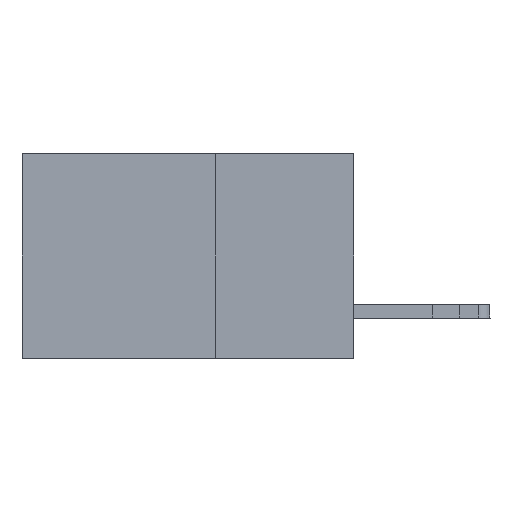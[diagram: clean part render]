
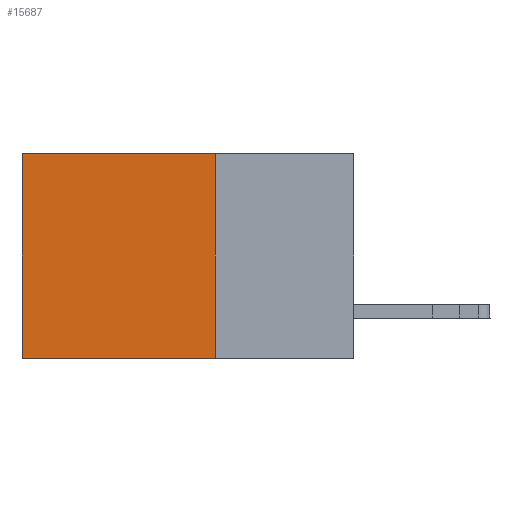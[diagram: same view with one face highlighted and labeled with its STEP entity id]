
A CAD part, left-side view. The second image highlights one B-rep face of the part: STEP entity #15687.
In plain terms, the highlighted planar face has unit normal (-1, 0, 0).
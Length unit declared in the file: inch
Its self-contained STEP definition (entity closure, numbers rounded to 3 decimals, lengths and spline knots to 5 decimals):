
#505 = VERTEX_POINT ( 'NONE', #20577 ) ;
#4275 = EDGE_CURVE ( 'NONE', #505, #10407, #23486, .T. ) ;
#4421 = DIRECTION ( 'NONE',  ( 0., 1., 0. ) ) ;
#5596 = FACE_OUTER_BOUND ( 'NONE', #11088, .T. ) ;
#7403 = AXIS2_PLACEMENT_3D ( 'NONE', #14359, #34404, #26019 ) ;
#7715 = ORIENTED_EDGE ( 'NONE', *, *, #18132, .F. ) ;
#10338 = CARTESIAN_POINT ( 'NONE',  ( 0.2875, 0.25, -0.37 ) ) ;
#10407 = VERTEX_POINT ( 'NONE', #10883 ) ;
#10883 = CARTESIAN_POINT ( 'NONE',  ( 0.2875, 0.6, -0.37 ) ) ;
#11088 = EDGE_LOOP ( 'NONE', ( #12563, #32563, #7715, #23462 ) ) ;
#11549 = CARTESIAN_POINT ( 'NONE',  ( 0.2875, 0.25, 0. ) ) ;
#12401 = VECTOR ( 'NONE', #32161, 39.37008 ) ;
#12563 = ORIENTED_EDGE ( 'NONE', *, *, #4275, .T. ) ;
#13032 = VERTEX_POINT ( 'NONE', #18797 ) ;
#14359 = CARTESIAN_POINT ( 'NONE',  ( 0.2875, 0.25, 0. ) ) ;
#15687 = ADVANCED_FACE ( 'NONE', ( #5596 ), #20102, .F. ) ;
#15986 = VERTEX_POINT ( 'NONE', #10338 ) ;
#16618 = CARTESIAN_POINT ( 'NONE',  ( 0.2875, 0.25, -0.37 ) ) ;
#16672 = LINE ( 'NONE', #22591, #27240 ) ;
#18132 = EDGE_CURVE ( 'NONE', #13032, #15986, #23574, .T. ) ;
#18797 = CARTESIAN_POINT ( 'NONE',  ( 0.2875, 0.25, 0. ) ) ;
#20102 = PLANE ( 'NONE',  #7403 ) ;
#20577 = CARTESIAN_POINT ( 'NONE',  ( 0.2875, 0.6, 0. ) ) ;
#22591 = CARTESIAN_POINT ( 'NONE',  ( 0.2875, 0.25, 0. ) ) ;
#23462 = ORIENTED_EDGE ( 'NONE', *, *, #34914, .T. ) ;
#23486 = LINE ( 'NONE', #32448, #32926 ) ;
#23574 = LINE ( 'NONE', #11549, #12401 ) ;
#26019 = DIRECTION ( 'NONE',  ( 0., 0., -1. ) ) ;
#26293 = VECTOR ( 'NONE', #4421, 39.37008 ) ;
#26782 = EDGE_CURVE ( 'NONE', #15986, #10407, #30544, .T. ) ;
#26911 = DIRECTION ( 'NONE',  ( 0., 0., -1. ) ) ;
#27240 = VECTOR ( 'NONE', #34008, 39.37008 ) ;
#30544 = LINE ( 'NONE', #16618, #26293 ) ;
#32161 = DIRECTION ( 'NONE',  ( 0., 0., -1. ) ) ;
#32448 = CARTESIAN_POINT ( 'NONE',  ( 0.2875, 0.6, 0. ) ) ;
#32563 = ORIENTED_EDGE ( 'NONE', *, *, #26782, .F. ) ;
#32926 = VECTOR ( 'NONE', #26911, 39.37008 ) ;
#34008 = DIRECTION ( 'NONE',  ( 0., 1., 0. ) ) ;
#34404 = DIRECTION ( 'NONE',  ( 1., 0., 0. ) ) ;
#34914 = EDGE_CURVE ( 'NONE', #13032, #505, #16672, .T. ) ;
